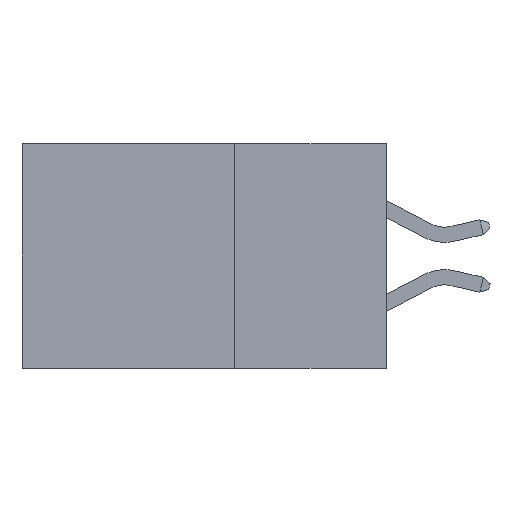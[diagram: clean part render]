
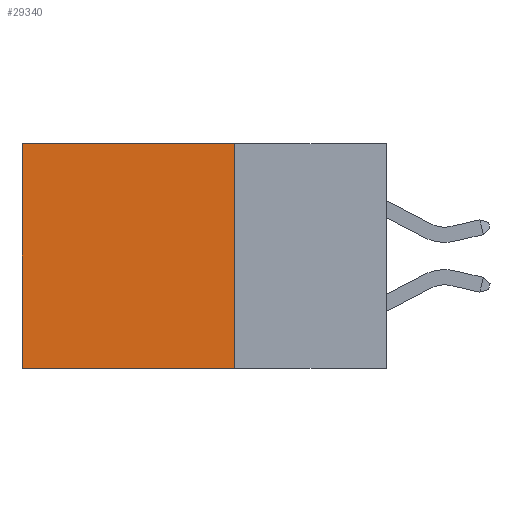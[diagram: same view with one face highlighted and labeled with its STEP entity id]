
A CAD part, left-side view. The second image highlights one B-rep face of the part: STEP entity #29340.
In plain terms, the highlighted planar face has unit normal (-1, 0, 0).
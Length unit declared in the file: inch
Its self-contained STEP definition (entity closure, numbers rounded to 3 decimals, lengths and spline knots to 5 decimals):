
#418 = CARTESIAN_POINT ( 'NONE',  ( 0.298, 0.25, 0. ) ) ;
#1386 = VECTOR ( 'NONE', #21370, 39.37008 ) ;
#1956 = CARTESIAN_POINT ( 'NONE',  ( 0.298, 0.6, 0. ) ) ;
#2816 = AXIS2_PLACEMENT_3D ( 'NONE', #15534, #22362, #19684 ) ;
#3119 = VECTOR ( 'NONE', #27554, 39.37008 ) ;
#3731 = LINE ( 'NONE', #418, #24882 ) ;
#3735 = EDGE_CURVE ( 'NONE', #10177, #21415, #11557, .T. ) ;
#3853 = ORIENTED_EDGE ( 'NONE', *, *, #6029, .F. ) ;
#3921 = EDGE_CURVE ( 'NONE', #17697, #10177, #11175, .T. ) ;
#4930 = CARTESIAN_POINT ( 'NONE',  ( 0.298, 0.6, 0. ) ) ;
#6029 = EDGE_CURVE ( 'NONE', #17697, #17184, #3731, .T. ) ;
#10177 = VERTEX_POINT ( 'NONE', #1956 ) ;
#11175 = LINE ( 'NONE', #29916, #3119 ) ;
#11557 = LINE ( 'NONE', #4930, #13728 ) ;
#13110 = PLANE ( 'NONE',  #2816 ) ;
#13728 = VECTOR ( 'NONE', #16717, 39.37008 ) ;
#15534 = CARTESIAN_POINT ( 'NONE',  ( 0.298, 0.25, 0. ) ) ;
#16308 = CARTESIAN_POINT ( 'NONE',  ( 0.298, 0.25, -0.37 ) ) ;
#16717 = DIRECTION ( 'NONE',  ( 0., 0., -1. ) ) ;
#17007 = EDGE_CURVE ( 'NONE', #17184, #21415, #29099, .T. ) ;
#17184 = VERTEX_POINT ( 'NONE', #16308 ) ;
#17697 = VERTEX_POINT ( 'NONE', #22421 ) ;
#19684 = DIRECTION ( 'NONE',  ( 0., 0., -1. ) ) ;
#20165 = EDGE_LOOP ( 'NONE', ( #24188, #26305, #3853, #21955 ) ) ;
#21370 = DIRECTION ( 'NONE',  ( 0., 1., 0. ) ) ;
#21415 = VERTEX_POINT ( 'NONE', #21999 ) ;
#21955 = ORIENTED_EDGE ( 'NONE', *, *, #3921, .T. ) ;
#21999 = CARTESIAN_POINT ( 'NONE',  ( 0.298, 0.6, -0.37 ) ) ;
#22362 = DIRECTION ( 'NONE',  ( 1., 0., 0. ) ) ;
#22421 = CARTESIAN_POINT ( 'NONE',  ( 0.298, 0.25, 0. ) ) ;
#22564 = CARTESIAN_POINT ( 'NONE',  ( 0.298, 0.25, -0.37 ) ) ;
#24188 = ORIENTED_EDGE ( 'NONE', *, *, #3735, .T. ) ;
#24882 = VECTOR ( 'NONE', #26084, 39.37008 ) ;
#26084 = DIRECTION ( 'NONE',  ( 0., 0., -1. ) ) ;
#26305 = ORIENTED_EDGE ( 'NONE', *, *, #17007, .F. ) ;
#27554 = DIRECTION ( 'NONE',  ( 0., 1., 0. ) ) ;
#29014 = FACE_OUTER_BOUND ( 'NONE', #20165, .T. ) ;
#29099 = LINE ( 'NONE', #22564, #1386 ) ;
#29340 = ADVANCED_FACE ( 'NONE', ( #29014 ), #13110, .F. ) ;
#29916 = CARTESIAN_POINT ( 'NONE',  ( 0.298, 0.25, 0. ) ) ;
